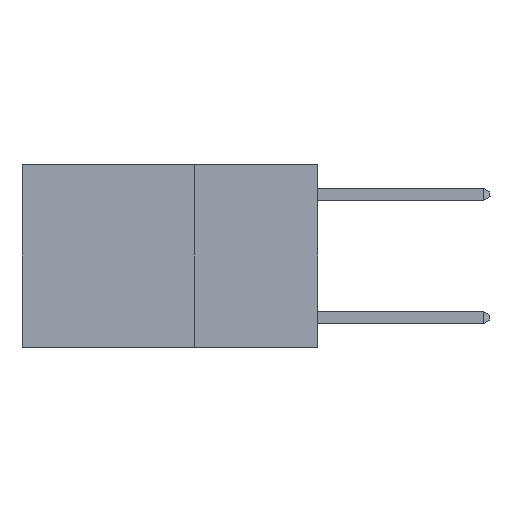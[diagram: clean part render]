
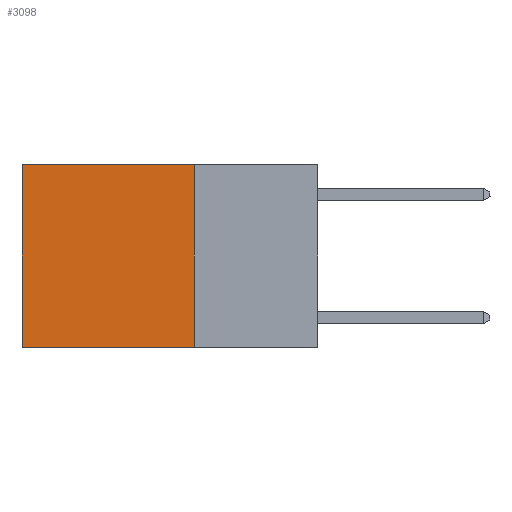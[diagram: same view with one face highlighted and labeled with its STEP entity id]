
A CAD part, left-side view. The second image highlights one B-rep face of the part: STEP entity #3098.
In plain terms, the highlighted planar face has unit normal (-1, 0, 0).
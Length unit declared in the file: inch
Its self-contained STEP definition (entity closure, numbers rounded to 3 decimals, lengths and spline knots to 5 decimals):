
#130 = ORIENTED_EDGE ( 'NONE', *, *, #5127, .F. ) ;
#157 = EDGE_CURVE ( 'NONE', #4335, #5419, #2140, .T. ) ;
#160 = ORIENTED_EDGE ( 'NONE', *, *, #157, .T. ) ;
#408 = VECTOR ( 'NONE', #6994, 39.37008 ) ;
#778 = LINE ( 'NONE', #8134, #2751 ) ;
#1322 = DIRECTION ( 'NONE',  ( 0., 0., -1. ) ) ;
#1333 = CARTESIAN_POINT ( 'NONE',  ( 0.2625, 0.25, 0. ) ) ;
#1397 = CARTESIAN_POINT ( 'NONE',  ( 0.2625, 0.6, 0. ) ) ;
#1564 = EDGE_LOOP ( 'NONE', ( #8927, #9047, #130, #160 ) ) ;
#2140 = LINE ( 'NONE', #3618, #408 ) ;
#2751 = VECTOR ( 'NONE', #4729, 39.37008 ) ;
#3098 = ADVANCED_FACE ( 'NONE', ( #6753 ), #8976, .F. ) ;
#3618 = CARTESIAN_POINT ( 'NONE',  ( 0.2625, 0.25, 0. ) ) ;
#4060 = DIRECTION ( 'NONE',  ( 1., 0., 0. ) ) ;
#4335 = VERTEX_POINT ( 'NONE', #6425 ) ;
#4455 = VECTOR ( 'NONE', #1322, 39.37008 ) ;
#4729 = DIRECTION ( 'NONE',  ( 0., 1., 0. ) ) ;
#4949 = CARTESIAN_POINT ( 'NONE',  ( 0.2625, 0.6, -0.37 ) ) ;
#5064 = AXIS2_PLACEMENT_3D ( 'NONE', #6468, #4060, #5715 ) ;
#5127 = EDGE_CURVE ( 'NONE', #4335, #6237, #8093, .T. ) ;
#5309 = VECTOR ( 'NONE', #5749, 39.37008 ) ;
#5419 = VERTEX_POINT ( 'NONE', #8628 ) ;
#5715 = DIRECTION ( 'NONE',  ( 0., 0., -1. ) ) ;
#5719 = LINE ( 'NONE', #1397, #5309 ) ;
#5749 = DIRECTION ( 'NONE',  ( 0., 0., -1. ) ) ;
#6197 = VERTEX_POINT ( 'NONE', #4949 ) ;
#6237 = VERTEX_POINT ( 'NONE', #8372 ) ;
#6425 = CARTESIAN_POINT ( 'NONE',  ( 0.2625, 0.25, 0. ) ) ;
#6468 = CARTESIAN_POINT ( 'NONE',  ( 0.2625, 0.25, 0. ) ) ;
#6753 = FACE_OUTER_BOUND ( 'NONE', #1564, .T. ) ;
#6994 = DIRECTION ( 'NONE',  ( 0., 1., 0. ) ) ;
#7081 = EDGE_CURVE ( 'NONE', #5419, #6197, #5719, .T. ) ;
#8093 = LINE ( 'NONE', #1333, #4455 ) ;
#8134 = CARTESIAN_POINT ( 'NONE',  ( 0.2625, 0.25, -0.37 ) ) ;
#8372 = CARTESIAN_POINT ( 'NONE',  ( 0.2625, 0.25, -0.37 ) ) ;
#8628 = CARTESIAN_POINT ( 'NONE',  ( 0.2625, 0.6, 0. ) ) ;
#8927 = ORIENTED_EDGE ( 'NONE', *, *, #7081, .T. ) ;
#8976 = PLANE ( 'NONE',  #5064 ) ;
#8990 = EDGE_CURVE ( 'NONE', #6237, #6197, #778, .T. ) ;
#9047 = ORIENTED_EDGE ( 'NONE', *, *, #8990, .F. ) ;
